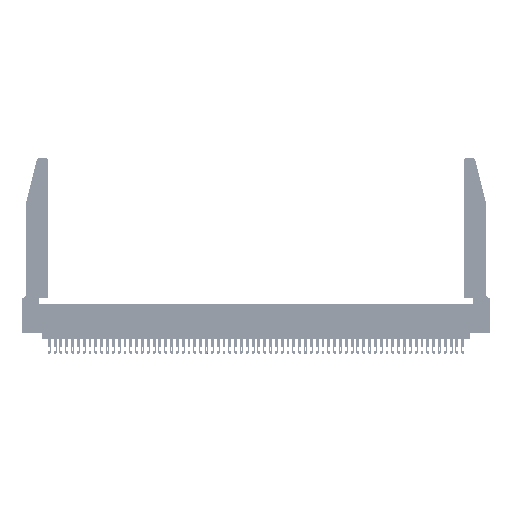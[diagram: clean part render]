
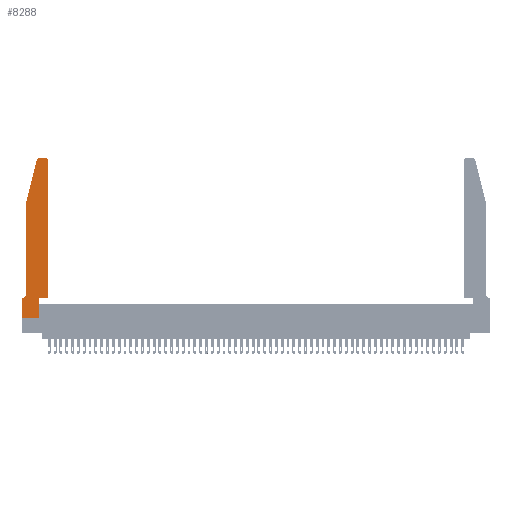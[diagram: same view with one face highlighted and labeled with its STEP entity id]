
A CAD part, top view. The second image highlights one B-rep face of the part: STEP entity #8288.
In plain terms, the highlighted planar face has unit normal (0, 0, 1).
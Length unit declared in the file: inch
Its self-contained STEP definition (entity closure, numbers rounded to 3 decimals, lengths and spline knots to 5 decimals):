
#998 = VECTOR ( 'NONE', #47400, 39.37008 ) ;
#1654 = VECTOR ( 'NONE', #53852, 39.37008 ) ;
#1682 = DIRECTION ( 'NONE',  ( 1., 0., 0. ) ) ;
#2058 = DIRECTION ( 'NONE',  ( 0., -1., 0. ) ) ;
#3355 = LINE ( 'NONE', #54811, #10281 ) ;
#4883 = DIRECTION ( 'NONE',  ( -1., 0., 0. ) ) ;
#5076 = CARTESIAN_POINT ( 'NONE',  ( 0.0755, 0.35, 0.37 ) ) ;
#6203 = VERTEX_POINT ( 'NONE', #17749 ) ;
#7513 = AXIS2_PLACEMENT_3D ( 'NONE', #16103, #42975, #38121 ) ;
#8288 = ADVANCED_FACE ( 'NONE', ( #18503 ), #28966, .T. ) ;
#8685 = CARTESIAN_POINT ( 'NONE',  ( 0.284, 2.75, 0.37 ) ) ;
#9052 = ORIENTED_EDGE ( 'NONE', *, *, #46725, .T. ) ;
#9836 = EDGE_CURVE ( 'NONE', #39868, #10959, #49525, .T. ) ;
#10281 = VECTOR ( 'NONE', #54620, 39.37008 ) ;
#10544 = EDGE_CURVE ( 'NONE', #6203, #40142, #55674, .T. ) ;
#10748 = VERTEX_POINT ( 'NONE', #13762 ) ;
#10803 = CARTESIAN_POINT ( 'NONE',  ( 0., 0.35, 0.37 ) ) ;
#10829 = EDGE_CURVE ( 'NONE', #30894, #10748, #41790, .T. ) ;
#10959 = VERTEX_POINT ( 'NONE', #23620 ) ;
#11521 = CARTESIAN_POINT ( 'NONE',  ( 0.0755, 2., 0.37 ) ) ;
#12275 = CARTESIAN_POINT ( 'NONE',  ( 0., 0., 0.37 ) ) ;
#12730 = VECTOR ( 'NONE', #4883, 39.37008 ) ;
#13175 = CARTESIAN_POINT ( 'NONE',  ( 0.0755, 0.42, 0.37 ) ) ;
#13230 = AXIS2_PLACEMENT_3D ( 'NONE', #10803, #54684, #41700 ) ;
#13702 = EDGE_CURVE ( 'NONE', #10959, #54348, #13995, .T. ) ;
#13762 = CARTESIAN_POINT ( 'NONE',  ( 0., 0.35, 0.37 ) ) ;
#13995 = LINE ( 'NONE', #54903, #27873 ) ;
#14721 = VERTEX_POINT ( 'NONE', #31167 ) ;
#14822 = CARTESIAN_POINT ( 'NONE',  ( 0.0055, 0.35, 0.37 ) ) ;
#14877 = ORIENTED_EDGE ( 'NONE', *, *, #52252, .T. ) ;
#15453 = DIRECTION ( 'NONE',  ( -1., 0., 0. ) ) ;
#16003 = DIRECTION ( 'NONE',  ( -0.239, -0.971, 0. ) ) ;
#16103 = CARTESIAN_POINT ( 'NONE',  ( 0.284, 2.72, 0.37 ) ) ;
#16519 = DIRECTION ( 'NONE',  ( 0., -1., 0. ) ) ;
#17749 = CARTESIAN_POINT ( 'NONE',  ( 0., 0., 0.37 ) ) ;
#18247 = CARTESIAN_POINT ( 'NONE',  ( 0.2865, 0.35, 0.37 ) ) ;
#18503 = FACE_OUTER_BOUND ( 'NONE', #55897, .T. ) ;
#19146 = VERTEX_POINT ( 'NONE', #19465 ) ;
#19465 = CARTESIAN_POINT ( 'NONE',  ( 0.2865, 0.35, 0.37 ) ) ;
#19632 = EDGE_CURVE ( 'NONE', #40827, #39868, #3355, .T. ) ;
#19906 = CARTESIAN_POINT ( 'NONE',  ( 0.4505, 2.72, 0.37 ) ) ;
#20109 = CIRCLE ( 'NONE', #25935, 0.07 ) ;
#21289 = VECTOR ( 'NONE', #50266, 39.37008 ) ;
#22484 = CARTESIAN_POINT ( 'NONE',  ( 0.0055, 0.42, 0.37 ) ) ;
#23620 = CARTESIAN_POINT ( 'NONE',  ( 0.4205, 2.75, 0.37 ) ) ;
#25278 = ORIENTED_EDGE ( 'NONE', *, *, #9836, .T. ) ;
#25935 = AXIS2_PLACEMENT_3D ( 'NONE', #22484, #27143, #35830 ) ;
#26226 = ORIENTED_EDGE ( 'NONE', *, *, #47810, .T. ) ;
#27143 = DIRECTION ( 'NONE',  ( 0., 0., -1. ) ) ;
#27263 = VERTEX_POINT ( 'NONE', #49655 ) ;
#27873 = VECTOR ( 'NONE', #15453, 39.37008 ) ;
#28180 = DIRECTION ( 'NONE',  ( 0., 0., 1. ) ) ;
#28966 = PLANE ( 'NONE',  #13230 ) ;
#30861 = ORIENTED_EDGE ( 'NONE', *, *, #10829, .T. ) ;
#30894 = VERTEX_POINT ( 'NONE', #14822 ) ;
#31167 = CARTESIAN_POINT ( 'NONE',  ( 0.25487, 2.72718, 0.37 ) ) ;
#32432 = LINE ( 'NONE', #33593, #35873 ) ;
#33032 = LINE ( 'NONE', #55473, #21289 ) ;
#33593 = CARTESIAN_POINT ( 'NONE',  ( 0.0755, 2., 0.37 ) ) ;
#33870 = EDGE_CURVE ( 'NONE', #10748, #6203, #48967, .T. ) ;
#34144 = EDGE_CURVE ( 'NONE', #19146, #40827, #33032, .T. ) ;
#35495 = CIRCLE ( 'NONE', #7513, 0.03 ) ;
#35830 = DIRECTION ( 'NONE',  ( -1., 0., 0. ) ) ;
#35873 = VECTOR ( 'NONE', #16003, 39.37008 ) ;
#36566 = EDGE_CURVE ( 'NONE', #54348, #14721, #35495, .T. ) ;
#36920 = LINE ( 'NONE', #18247, #1654 ) ;
#37219 = ORIENTED_EDGE ( 'NONE', *, *, #10544, .T. ) ;
#38121 = DIRECTION ( 'NONE',  ( 1., 0., 0. ) ) ;
#38130 = CARTESIAN_POINT ( 'NONE',  ( 0., 0., 0.37 ) ) ;
#38503 = ORIENTED_EDGE ( 'NONE', *, *, #13702, .T. ) ;
#39293 = VECTOR ( 'NONE', #16519, 39.37008 ) ;
#39868 = VERTEX_POINT ( 'NONE', #19906 ) ;
#40142 = VERTEX_POINT ( 'NONE', #52887 ) ;
#40827 = VERTEX_POINT ( 'NONE', #45235 ) ;
#41700 = DIRECTION ( 'NONE',  ( 1., 0., 0. ) ) ;
#41790 = LINE ( 'NONE', #5076, #12730 ) ;
#42525 = AXIS2_PLACEMENT_3D ( 'NONE', #46291, #28180, #1682 ) ;
#42975 = DIRECTION ( 'NONE',  ( 0., 0., 1. ) ) ;
#43272 = ORIENTED_EDGE ( 'NONE', *, *, #51659, .T. ) ;
#45235 = CARTESIAN_POINT ( 'NONE',  ( 0.4505, 0.35, 0.37 ) ) ;
#46291 = CARTESIAN_POINT ( 'NONE',  ( 0.4205, 2.72, 0.37 ) ) ;
#46540 = LINE ( 'NONE', #11521, #56939 ) ;
#46725 = EDGE_CURVE ( 'NONE', #56298, #30894, #20109, .T. ) ;
#47400 = DIRECTION ( 'NONE',  ( 1., 0., 0. ) ) ;
#47810 = EDGE_CURVE ( 'NONE', #14721, #27263, #32432, .T. ) ;
#48195 = ORIENTED_EDGE ( 'NONE', *, *, #33870, .T. ) ;
#48967 = LINE ( 'NONE', #12275, #39293 ) ;
#49203 = ORIENTED_EDGE ( 'NONE', *, *, #36566, .T. ) ;
#49525 = CIRCLE ( 'NONE', #42525, 0.03 ) ;
#49655 = CARTESIAN_POINT ( 'NONE',  ( 0.0755, 2., 0.37 ) ) ;
#50266 = DIRECTION ( 'NONE',  ( 1., 0., 0. ) ) ;
#51659 = EDGE_CURVE ( 'NONE', #40142, #19146, #36920, .T. ) ;
#52252 = EDGE_CURVE ( 'NONE', #27263, #56298, #46540, .T. ) ;
#52887 = CARTESIAN_POINT ( 'NONE',  ( 0.2865, 0., 0.37 ) ) ;
#53852 = DIRECTION ( 'NONE',  ( 0., 1., 0. ) ) ;
#54348 = VERTEX_POINT ( 'NONE', #8685 ) ;
#54620 = DIRECTION ( 'NONE',  ( 0., 1., 0. ) ) ;
#54684 = DIRECTION ( 'NONE',  ( 0., 0., 1. ) ) ;
#54811 = CARTESIAN_POINT ( 'NONE',  ( 0.4505, 0.35, 0.37 ) ) ;
#54903 = CARTESIAN_POINT ( 'NONE',  ( 0.2605, 2.75, 0.37 ) ) ;
#55119 = ORIENTED_EDGE ( 'NONE', *, *, #19632, .T. ) ;
#55473 = CARTESIAN_POINT ( 'NONE',  ( 0.4505, 0.35, 0.37 ) ) ;
#55602 = ORIENTED_EDGE ( 'NONE', *, *, #34144, .T. ) ;
#55674 = LINE ( 'NONE', #38130, #998 ) ;
#55897 = EDGE_LOOP ( 'NONE', ( #38503, #49203, #26226, #14877, #9052, #30861, #48195, #37219, #43272, #55602, #55119, #25278 ) ) ;
#56298 = VERTEX_POINT ( 'NONE', #13175 ) ;
#56939 = VECTOR ( 'NONE', #2058, 39.37008 ) ;
